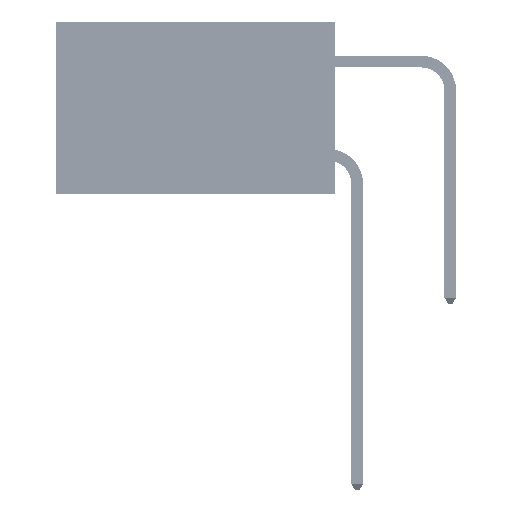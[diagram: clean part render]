
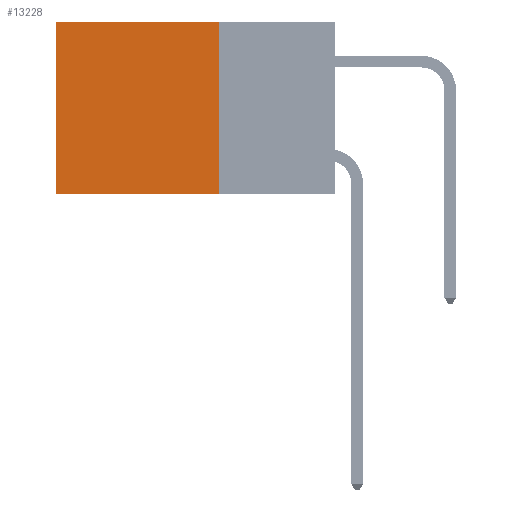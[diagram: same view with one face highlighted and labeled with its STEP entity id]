
A CAD part, left-side view. The second image highlights one B-rep face of the part: STEP entity #13228.
In plain terms, the highlighted planar face has unit normal (-1, 0, 0).
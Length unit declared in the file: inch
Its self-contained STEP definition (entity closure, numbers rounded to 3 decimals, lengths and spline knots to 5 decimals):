
#3477 = CARTESIAN_POINT ( 'NONE',  ( 0.2875, 0.6, 0. ) ) ;
#4753 = VERTEX_POINT ( 'NONE', #44835 ) ;
#6897 = EDGE_CURVE ( 'NONE', #26557, #38648, #15698, .T. ) ;
#8456 = ORIENTED_EDGE ( 'NONE', *, *, #45413, .F. ) ;
#11956 = EDGE_CURVE ( 'NONE', #4753, #42008, #28399, .T. ) ;
#12825 = DIRECTION ( 'NONE',  ( 0., 1., 0. ) ) ;
#13228 = ADVANCED_FACE ( 'NONE', ( #16118 ), #39950, .F. ) ;
#13676 = ORIENTED_EDGE ( 'NONE', *, *, #33463, .T. ) ;
#15698 = LINE ( 'NONE', #28476, #38341 ) ;
#16118 = FACE_OUTER_BOUND ( 'NONE', #20432, .T. ) ;
#17699 = VECTOR ( 'NONE', #19538, 39.37008 ) ;
#19538 = DIRECTION ( 'NONE',  ( 0., 1., 0. ) ) ;
#19638 = LINE ( 'NONE', #34987, #30983 ) ;
#20432 = EDGE_LOOP ( 'NONE', ( #13676, #38707, #8456, #36334 ) ) ;
#26557 = VERTEX_POINT ( 'NONE', #48663 ) ;
#27418 = AXIS2_PLACEMENT_3D ( 'NONE', #35520, #47499, #51731 ) ;
#28399 = LINE ( 'NONE', #51735, #17699 ) ;
#28476 = CARTESIAN_POINT ( 'NONE',  ( 0.2875, 0.25, -0.37 ) ) ;
#30983 = VECTOR ( 'NONE', #43274, 39.37008 ) ;
#33463 = EDGE_CURVE ( 'NONE', #42008, #38648, #34717, .T. ) ;
#34717 = LINE ( 'NONE', #3477, #51065 ) ;
#34987 = CARTESIAN_POINT ( 'NONE',  ( 0.2875, 0.25, 0. ) ) ;
#35520 = CARTESIAN_POINT ( 'NONE',  ( 0.2875, 0.25, 0. ) ) ;
#36334 = ORIENTED_EDGE ( 'NONE', *, *, #11956, .T. ) ;
#38139 = CARTESIAN_POINT ( 'NONE',  ( 0.2875, 0.6, 0. ) ) ;
#38341 = VECTOR ( 'NONE', #12825, 39.37008 ) ;
#38648 = VERTEX_POINT ( 'NONE', #44699 ) ;
#38707 = ORIENTED_EDGE ( 'NONE', *, *, #6897, .F. ) ;
#39950 = PLANE ( 'NONE',  #27418 ) ;
#39965 = DIRECTION ( 'NONE',  ( 0., 0., -1. ) ) ;
#42008 = VERTEX_POINT ( 'NONE', #38139 ) ;
#43274 = DIRECTION ( 'NONE',  ( 0., 0., -1. ) ) ;
#44699 = CARTESIAN_POINT ( 'NONE',  ( 0.2875, 0.6, -0.37 ) ) ;
#44835 = CARTESIAN_POINT ( 'NONE',  ( 0.2875, 0.25, 0. ) ) ;
#45413 = EDGE_CURVE ( 'NONE', #4753, #26557, #19638, .T. ) ;
#47499 = DIRECTION ( 'NONE',  ( 1., 0., 0. ) ) ;
#48663 = CARTESIAN_POINT ( 'NONE',  ( 0.2875, 0.25, -0.37 ) ) ;
#51065 = VECTOR ( 'NONE', #39965, 39.37008 ) ;
#51731 = DIRECTION ( 'NONE',  ( 0., 0., -1. ) ) ;
#51735 = CARTESIAN_POINT ( 'NONE',  ( 0.2875, 0.25, 0. ) ) ;
